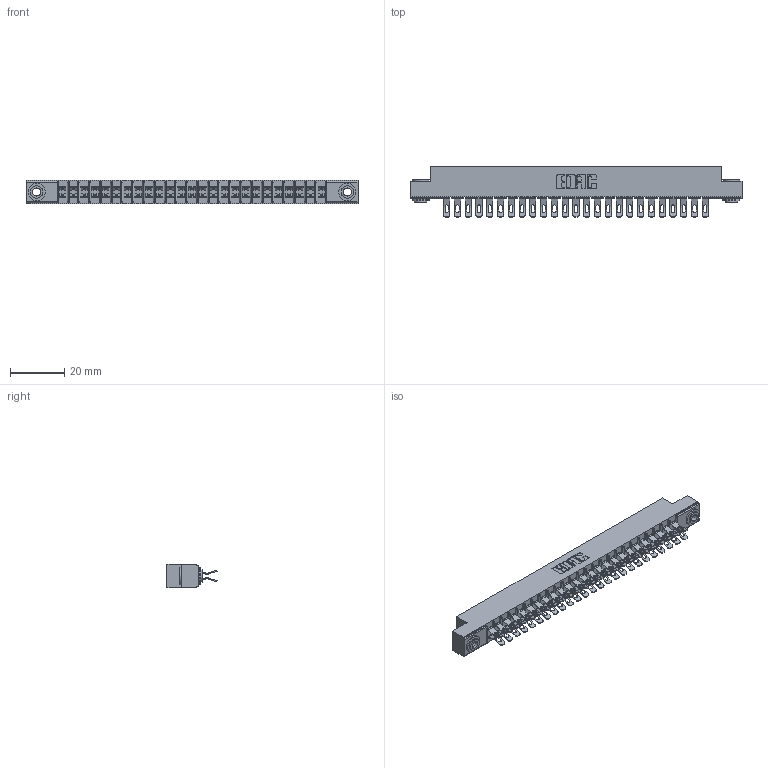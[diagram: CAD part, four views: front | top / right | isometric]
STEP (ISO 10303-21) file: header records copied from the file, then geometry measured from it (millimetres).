
FILE_DESCRIPTION (( 'STEP AP203' ), '1' );
FILE_NAME ('355-050-555-203.STEP', '2019-09-11T15:56:18', ( '' ), ( '' ), 'SwSTEP 2.0', 'SolidWorks 2016', '' );
FILE_SCHEMA (( 'CONFIG_CONTROL_DESIGN' ));
Length unit declared in the file: inch
Products named in the file (4): 345-250-002_345-250-002-102; 305-290-001_555; 305 Part_.156 Dia; 355-050-555-203
Assembly tree (53 placements, depth 2):
  355-050-555-203
    305 Part_.156 Dia
    305-290-001_555  x50
    345-250-002_345-250-002-102  x2
Bounding box: 122.07 x 18.41 x 8.71 mm (x, y, z)
Volume: 7796.4 mm3; surface area: 16004.8 mm2
Topology: 53 solids, 53 shells, 3468 faces, 10303 edges, 6730 vertices
Faces by surface type: plane 1692, cylinder 1668, sphere 100, cone 8
Entity records: 30827 total; most frequent: CARTESIAN_POINT 5100, ORIENTED_EDGE 5042, DIRECTION 4957, EDGE_CURVE 2521, VECTOR 1991, LINE 1991, VERTEX_POINT 1610, AXIS2_PLACEMENT_3D 1483
